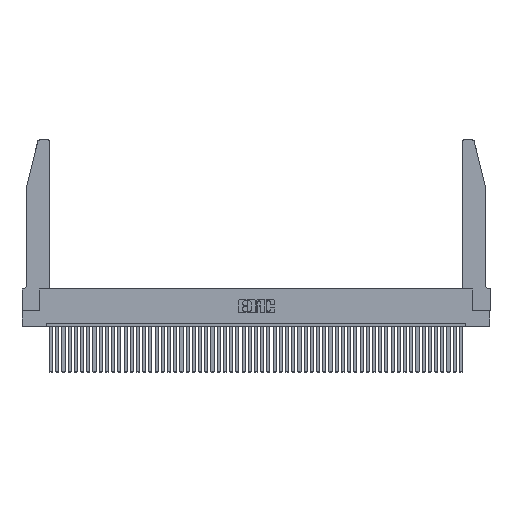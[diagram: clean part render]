
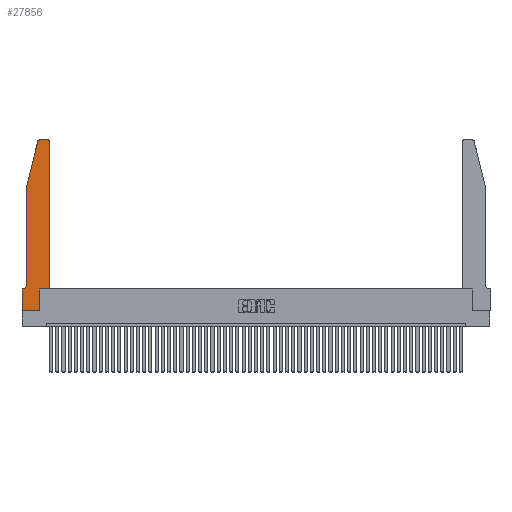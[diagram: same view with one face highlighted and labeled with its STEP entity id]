
A CAD part, top view. The second image highlights one B-rep face of the part: STEP entity #27856.
In plain terms, the highlighted planar face has unit normal (0, 0, 1).
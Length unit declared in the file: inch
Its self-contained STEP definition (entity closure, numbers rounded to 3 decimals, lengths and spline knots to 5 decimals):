
#978 = DIRECTION ( 'NONE',  ( -1., 0., 0. ) ) ;
#1142 = VECTOR ( 'NONE', #978, 39.37008 ) ;
#2249 = VECTOR ( 'NONE', #10376, 39.37008 ) ;
#2592 = CIRCLE ( 'NONE', #25088, 0.03 ) ;
#2932 = EDGE_LOOP ( 'NONE', ( #46740, #10741, #42993, #24191, #14964, #19663, #17271, #14829, #21350, #27426, #25299, #31428 ) ) ;
#3758 = VERTEX_POINT ( 'NONE', #9805 ) ;
#3976 = EDGE_CURVE ( 'NONE', #48967, #28878, #14237, .T. ) ;
#3981 = DIRECTION ( 'NONE',  ( 0., 0., -1. ) ) ;
#5730 = EDGE_CURVE ( 'NONE', #51020, #3758, #33952, .T. ) ;
#6852 = CARTESIAN_POINT ( 'NONE',  ( 0., 0.35, 0.37 ) ) ;
#6978 = VERTEX_POINT ( 'NONE', #25365 ) ;
#7505 = CARTESIAN_POINT ( 'NONE',  ( 0.0755, 2., 0.37 ) ) ;
#9551 = EDGE_CURVE ( 'NONE', #22924, #42238, #51527, .T. ) ;
#9634 = VECTOR ( 'NONE', #10012, 39.37008 ) ;
#9663 = EDGE_CURVE ( 'NONE', #21440, #51404, #40761, .T. ) ;
#9805 = CARTESIAN_POINT ( 'NONE',  ( 0.0755, 0.42, 0.37 ) ) ;
#10012 = DIRECTION ( 'NONE',  ( 0., 1., 0. ) ) ;
#10085 = CARTESIAN_POINT ( 'NONE',  ( 0.2865, 0.35, 0.37 ) ) ;
#10376 = DIRECTION ( 'NONE',  ( 0., -1., 0. ) ) ;
#10470 = DIRECTION ( 'NONE',  ( 1., 0., 0. ) ) ;
#10741 = ORIENTED_EDGE ( 'NONE', *, *, #47116, .T. ) ;
#11617 = CIRCLE ( 'NONE', #36415, 0.07 ) ;
#11732 = DIRECTION ( 'NONE',  ( 0., 0., 1. ) ) ;
#12657 = VECTOR ( 'NONE', #38310, 39.37008 ) ;
#13009 = DIRECTION ( 'NONE',  ( 1., 0., 0. ) ) ;
#13424 = FACE_OUTER_BOUND ( 'NONE', #2932, .T. ) ;
#13635 = CARTESIAN_POINT ( 'NONE',  ( 0.4505, 0.35, 0.37 ) ) ;
#14237 = LINE ( 'NONE', #29289, #1142 ) ;
#14829 = ORIENTED_EDGE ( 'NONE', *, *, #41105, .T. ) ;
#14964 = ORIENTED_EDGE ( 'NONE', *, *, #36753, .T. ) ;
#15754 = CARTESIAN_POINT ( 'NONE',  ( 0.4505, 0.35, 0.37 ) ) ;
#17161 = CARTESIAN_POINT ( 'NONE',  ( 0.284, 2.75, 0.37 ) ) ;
#17181 = EDGE_CURVE ( 'NONE', #42238, #21440, #49443, .T. ) ;
#17251 = LINE ( 'NONE', #38497, #20376 ) ;
#17271 = ORIENTED_EDGE ( 'NONE', *, *, #44114, .T. ) ;
#18502 = CARTESIAN_POINT ( 'NONE',  ( 0.0055, 0.42, 0.37 ) ) ;
#18957 = CARTESIAN_POINT ( 'NONE',  ( 0.4505, 0.35, 0.37 ) ) ;
#19663 = ORIENTED_EDGE ( 'NONE', *, *, #28691, .T. ) ;
#19863 = CARTESIAN_POINT ( 'NONE',  ( 0., 0., 0.37 ) ) ;
#20015 = AXIS2_PLACEMENT_3D ( 'NONE', #35585, #11732, #51659 ) ;
#20376 = VECTOR ( 'NONE', #22977, 39.37008 ) ;
#20448 = VERTEX_POINT ( 'NONE', #22859 ) ;
#21247 = CARTESIAN_POINT ( 'NONE',  ( 0.2865, 0.35, 0.37 ) ) ;
#21350 = ORIENTED_EDGE ( 'NONE', *, *, #9551, .T. ) ;
#21440 = VERTEX_POINT ( 'NONE', #13635 ) ;
#22859 = CARTESIAN_POINT ( 'NONE',  ( 0.0055, 0.35, 0.37 ) ) ;
#22924 = VERTEX_POINT ( 'NONE', #38873 ) ;
#22977 = DIRECTION ( 'NONE',  ( 0., -1., 0. ) ) ;
#23405 = CARTESIAN_POINT ( 'NONE',  ( 0.4205, 2.75, 0.37 ) ) ;
#24191 = ORIENTED_EDGE ( 'NONE', *, *, #5730, .T. ) ;
#25088 = AXIS2_PLACEMENT_3D ( 'NONE', #28515, #44921, #13009 ) ;
#25299 = ORIENTED_EDGE ( 'NONE', *, *, #9663, .T. ) ;
#25365 = CARTESIAN_POINT ( 'NONE',  ( 0.25487, 2.72718, 0.37 ) ) ;
#27426 = ORIENTED_EDGE ( 'NONE', *, *, #17181, .T. ) ;
#27711 = VECTOR ( 'NONE', #32425, 39.37008 ) ;
#27856 = ADVANCED_FACE ( 'NONE', ( #13424 ), #36015, .T. ) ;
#28002 = DIRECTION ( 'NONE',  ( 1., 0., 0. ) ) ;
#28515 = CARTESIAN_POINT ( 'NONE',  ( 0.4205, 2.72, 0.37 ) ) ;
#28691 = EDGE_CURVE ( 'NONE', #20448, #49523, #49492, .T. ) ;
#28878 = VERTEX_POINT ( 'NONE', #17161 ) ;
#29289 = CARTESIAN_POINT ( 'NONE',  ( 0.2605, 2.75, 0.37 ) ) ;
#29589 = LINE ( 'NONE', #46346, #31542 ) ;
#31428 = ORIENTED_EDGE ( 'NONE', *, *, #38320, .T. ) ;
#31542 = VECTOR ( 'NONE', #40887, 39.37008 ) ;
#32425 = DIRECTION ( 'NONE',  ( 0., 1., 0. ) ) ;
#33218 = CIRCLE ( 'NONE', #20015, 0.03 ) ;
#33671 = VECTOR ( 'NONE', #43170, 39.37008 ) ;
#33952 = LINE ( 'NONE', #34181, #2249 ) ;
#34181 = CARTESIAN_POINT ( 'NONE',  ( 0.0755, 2., 0.37 ) ) ;
#34635 = CARTESIAN_POINT ( 'NONE',  ( 0.0755, 0.35, 0.37 ) ) ;
#35399 = CARTESIAN_POINT ( 'NONE',  ( 0.0755, 2., 0.37 ) ) ;
#35585 = CARTESIAN_POINT ( 'NONE',  ( 0.284, 2.72, 0.37 ) ) ;
#36015 = PLANE ( 'NONE',  #45515 ) ;
#36415 = AXIS2_PLACEMENT_3D ( 'NONE', #18502, #3981, #39295 ) ;
#36753 = EDGE_CURVE ( 'NONE', #3758, #20448, #11617, .T. ) ;
#37525 = VECTOR ( 'NONE', #10470, 39.37008 ) ;
#38310 = DIRECTION ( 'NONE',  ( -1., 0., 0. ) ) ;
#38320 = EDGE_CURVE ( 'NONE', #51404, #48967, #2592, .T. ) ;
#38497 = CARTESIAN_POINT ( 'NONE',  ( 0., 0., 0.37 ) ) ;
#38873 = CARTESIAN_POINT ( 'NONE',  ( 0.2865, 0., 0.37 ) ) ;
#39295 = DIRECTION ( 'NONE',  ( -1., 0., 0. ) ) ;
#40386 = DIRECTION ( 'NONE',  ( 0., 0., 1. ) ) ;
#40761 = LINE ( 'NONE', #15754, #27711 ) ;
#40887 = DIRECTION ( 'NONE',  ( 1., 0., 0. ) ) ;
#41105 = EDGE_CURVE ( 'NONE', #49039, #22924, #29589, .T. ) ;
#42238 = VERTEX_POINT ( 'NONE', #10085 ) ;
#42993 = ORIENTED_EDGE ( 'NONE', *, *, #48330, .T. ) ;
#43170 = DIRECTION ( 'NONE',  ( -0.239, -0.971, 0. ) ) ;
#44114 = EDGE_CURVE ( 'NONE', #49523, #49039, #17251, .T. ) ;
#44308 = LINE ( 'NONE', #7505, #33671 ) ;
#44921 = DIRECTION ( 'NONE',  ( 0., 0., 1. ) ) ;
#45515 = AXIS2_PLACEMENT_3D ( 'NONE', #48428, #40386, #28002 ) ;
#46346 = CARTESIAN_POINT ( 'NONE',  ( 0., 0., 0.37 ) ) ;
#46723 = CARTESIAN_POINT ( 'NONE',  ( 0.4505, 2.72, 0.37 ) ) ;
#46740 = ORIENTED_EDGE ( 'NONE', *, *, #3976, .T. ) ;
#47116 = EDGE_CURVE ( 'NONE', #28878, #6978, #33218, .T. ) ;
#48330 = EDGE_CURVE ( 'NONE', #6978, #51020, #44308, .T. ) ;
#48428 = CARTESIAN_POINT ( 'NONE',  ( 0., 0.35, 0.37 ) ) ;
#48967 = VERTEX_POINT ( 'NONE', #23405 ) ;
#49039 = VERTEX_POINT ( 'NONE', #19863 ) ;
#49443 = LINE ( 'NONE', #18957, #37525 ) ;
#49492 = LINE ( 'NONE', #34635, #12657 ) ;
#49523 = VERTEX_POINT ( 'NONE', #6852 ) ;
#51020 = VERTEX_POINT ( 'NONE', #35399 ) ;
#51404 = VERTEX_POINT ( 'NONE', #46723 ) ;
#51527 = LINE ( 'NONE', #21247, #9634 ) ;
#51659 = DIRECTION ( 'NONE',  ( 1., 0., 0. ) ) ;
